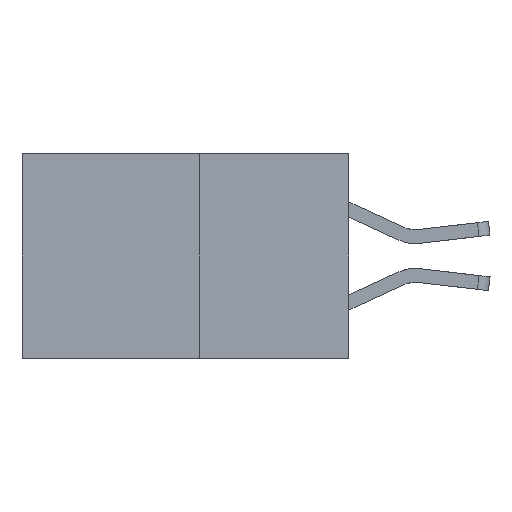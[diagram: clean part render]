
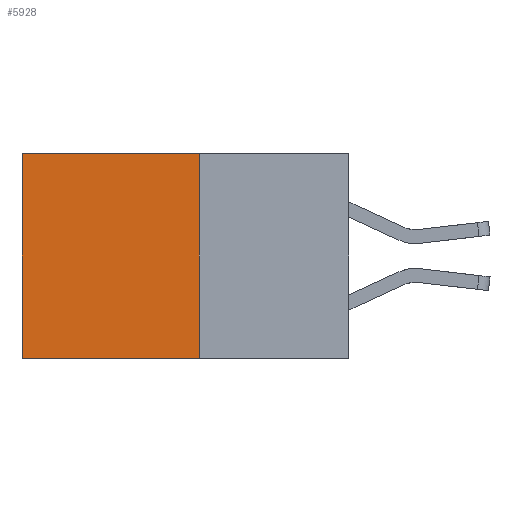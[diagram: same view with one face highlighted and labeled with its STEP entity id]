
A CAD part, left-side view. The second image highlights one B-rep face of the part: STEP entity #5928.
In plain terms, the highlighted planar face has unit normal (-1, 0, 0).
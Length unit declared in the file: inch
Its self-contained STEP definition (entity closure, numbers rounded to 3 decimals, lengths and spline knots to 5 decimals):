
#127 = EDGE_LOOP ( 'NONE', ( #3829, #8566, #2643, #7918 ) ) ;
#1086 = VERTEX_POINT ( 'NONE', #3716 ) ;
#1116 = EDGE_CURVE ( 'NONE', #1086, #6290, #1992, .T. ) ;
#1274 = CARTESIAN_POINT ( 'NONE',  ( 0.277, 0.27, -0.37 ) ) ;
#1479 = LINE ( 'NONE', #3059, #2328 ) ;
#1849 = EDGE_CURVE ( 'NONE', #1086, #2136, #1976, .T. ) ;
#1870 = CARTESIAN_POINT ( 'NONE',  ( 0.277, 0.59, -0.37 ) ) ;
#1976 = LINE ( 'NONE', #7425, #5423 ) ;
#1992 = LINE ( 'NONE', #2008, #3605 ) ;
#2008 = CARTESIAN_POINT ( 'NONE',  ( 0.277, 0.27, 0. ) ) ;
#2136 = VERTEX_POINT ( 'NONE', #1274 ) ;
#2159 = DIRECTION ( 'NONE',  ( 0., 1., 0. ) ) ;
#2328 = VECTOR ( 'NONE', #8573, 39.37008 ) ;
#2643 = ORIENTED_EDGE ( 'NONE', *, *, #1849, .F. ) ;
#3059 = CARTESIAN_POINT ( 'NONE',  ( 0.277, 0.27, -0.37 ) ) ;
#3306 = EDGE_CURVE ( 'NONE', #6290, #4829, #6554, .T. ) ;
#3605 = VECTOR ( 'NONE', #2159, 39.37008 ) ;
#3716 = CARTESIAN_POINT ( 'NONE',  ( 0.277, 0.27, 0. ) ) ;
#3723 = PLANE ( 'NONE',  #4270 ) ;
#3799 = CARTESIAN_POINT ( 'NONE',  ( 0.277, 0.59, -0.37 ) ) ;
#3829 = ORIENTED_EDGE ( 'NONE', *, *, #3306, .T. ) ;
#4270 = AXIS2_PLACEMENT_3D ( 'NONE', #5771, #8524, #4401 ) ;
#4401 = DIRECTION ( 'NONE',  ( 0., 0., -1. ) ) ;
#4829 = VERTEX_POINT ( 'NONE', #1870 ) ;
#4886 = FACE_OUTER_BOUND ( 'NONE', #127, .T. ) ;
#5151 = DIRECTION ( 'NONE',  ( 0., 0., -1. ) ) ;
#5423 = VECTOR ( 'NONE', #6357, 39.37008 ) ;
#5771 = CARTESIAN_POINT ( 'NONE',  ( 0.277, 0.27, -0.37 ) ) ;
#5928 = ADVANCED_FACE ( 'NONE', ( #4886 ), #3723, .F. ) ;
#6290 = VERTEX_POINT ( 'NONE', #8863 ) ;
#6357 = DIRECTION ( 'NONE',  ( 0., 0., -1. ) ) ;
#6359 = VECTOR ( 'NONE', #5151, 39.37008 ) ;
#6554 = LINE ( 'NONE', #3799, #6359 ) ;
#7425 = CARTESIAN_POINT ( 'NONE',  ( 0.277, 0.27, -0.37 ) ) ;
#7918 = ORIENTED_EDGE ( 'NONE', *, *, #1116, .T. ) ;
#8329 = EDGE_CURVE ( 'NONE', #2136, #4829, #1479, .T. ) ;
#8524 = DIRECTION ( 'NONE',  ( 1., 0., 0. ) ) ;
#8566 = ORIENTED_EDGE ( 'NONE', *, *, #8329, .F. ) ;
#8573 = DIRECTION ( 'NONE',  ( 0., 1., 0. ) ) ;
#8863 = CARTESIAN_POINT ( 'NONE',  ( 0.277, 0.59, 0. ) ) ;
